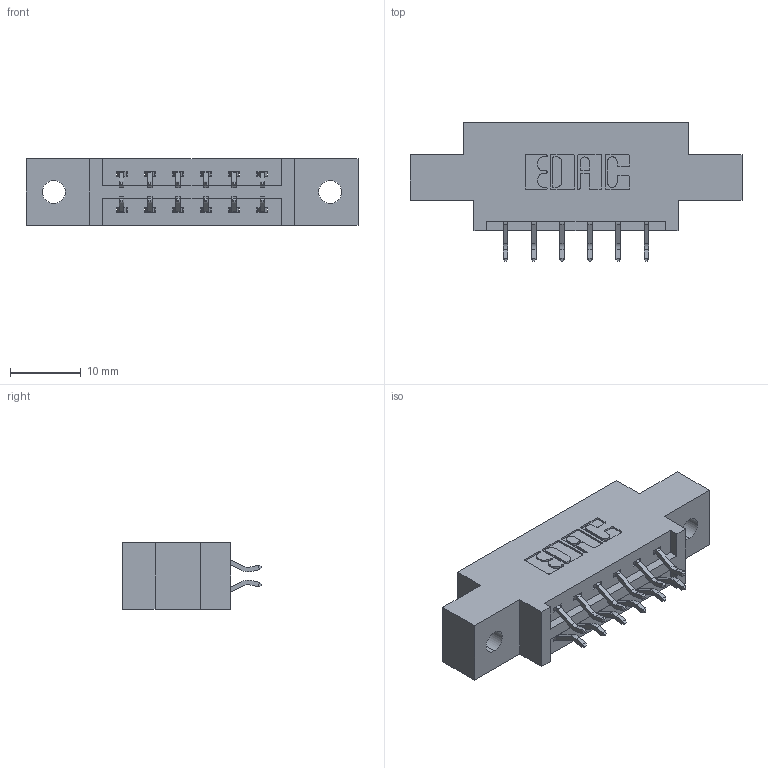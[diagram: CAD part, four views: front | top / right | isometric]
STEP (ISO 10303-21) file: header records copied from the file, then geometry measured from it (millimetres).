
FILE_DESCRIPTION (( 'STEP AP203' ), '1' );
FILE_NAME ('387-012-556-802.STEP', '2019-10-15T20:21:35', ( '' ), ( '' ), 'SwSTEP 2.0', 'SolidWorks 2016', '' );
FILE_SCHEMA (( 'CONFIG_CONTROL_DESIGN' ));
Length unit declared in the file: inch
Products named in the file (3): 337 Part_0.170 Offset - 0.128 Dia; 345-292-001_556 Tail; 387-012-556-802
Assembly tree (13 placements, depth 2):
  387-012-556-802
    337 Part_0.170 Offset - 0.128 Dia
    345-292-001_556 Tail  x12
Bounding box: 46.79 x 19.57 x 9.4 mm (x, y, z)
Volume: 4296.9 mm3; surface area: 4330.4 mm2
Topology: 13 solids, 13 shells, 838 faces, 2471 edges, 1630 vertices
Faces by surface type: plane 578, cylinder 260
Entity records: 9663 total; most frequent: CARTESIAN_POINT 1674, ORIENTED_EDGE 1598, DIRECTION 1479, EDGE_CURVE 799, VECTOR 663, LINE 663, VERTEX_POINT 530, AXIS2_PLACEMENT_3D 408
